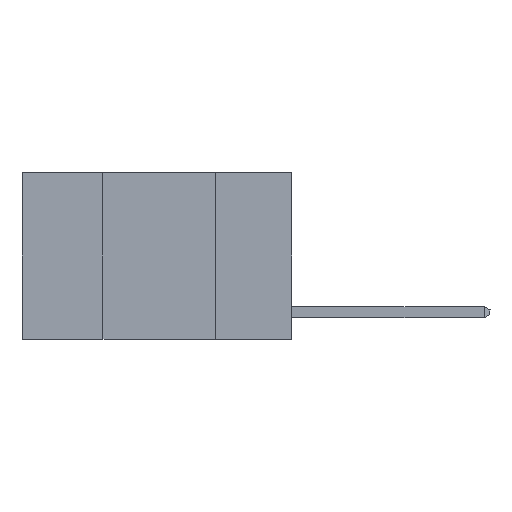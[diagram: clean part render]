
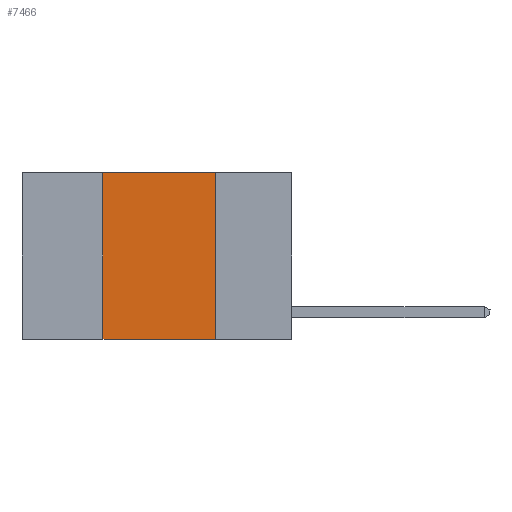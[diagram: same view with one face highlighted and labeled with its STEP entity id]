
A CAD part, left-side view. The second image highlights one B-rep face of the part: STEP entity #7466.
In plain terms, the highlighted planar face has unit normal (-1, 0, 0).
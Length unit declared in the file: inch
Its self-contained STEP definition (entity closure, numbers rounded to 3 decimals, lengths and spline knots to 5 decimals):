
#523 = CARTESIAN_POINT ( 'NONE',  ( 0., 0.42, -0.37 ) ) ;
#1208 = ORIENTED_EDGE ( 'NONE', *, *, #2267, .F. ) ;
#1470 = CARTESIAN_POINT ( 'NONE',  ( 0., 0.42, 0. ) ) ;
#2267 = EDGE_CURVE ( 'NONE', #13954, #2272, #3091, .T. ) ;
#2272 = VERTEX_POINT ( 'NONE', #8284 ) ;
#2611 = LINE ( 'NONE', #10808, #8658 ) ;
#3091 = LINE ( 'NONE', #8448, #12381 ) ;
#4083 = LINE ( 'NONE', #4106, #10171 ) ;
#4106 = CARTESIAN_POINT ( 'NONE',  ( 0., 0.42, 0. ) ) ;
#4417 = ORIENTED_EDGE ( 'NONE', *, *, #9108, .F. ) ;
#4813 = VECTOR ( 'NONE', #14393, 39.37008 ) ;
#4886 = DIRECTION ( 'NONE',  ( 0., 0., -1. ) ) ;
#5337 = DIRECTION ( 'NONE',  ( 0., 0., 1. ) ) ;
#5832 = CARTESIAN_POINT ( 'NONE',  ( 0., 0.17, -0.37 ) ) ;
#6704 = AXIS2_PLACEMENT_3D ( 'NONE', #9728, #12150, #4886 ) ;
#7096 = CARTESIAN_POINT ( 'NONE',  ( 0., 0.6, -0.37 ) ) ;
#7266 = PLANE ( 'NONE',  #6704 ) ;
#7336 = VERTEX_POINT ( 'NONE', #5832 ) ;
#7466 = ADVANCED_FACE ( 'NONE', ( #11537 ), #7266, .F. ) ;
#7810 = EDGE_LOOP ( 'NONE', ( #10499, #1208, #4417, #14109 ) ) ;
#8284 = CARTESIAN_POINT ( 'NONE',  ( 0., 0.17, 0. ) ) ;
#8317 = VERTEX_POINT ( 'NONE', #523 ) ;
#8444 = DIRECTION ( 'NONE',  ( 0., -1., 0. ) ) ;
#8448 = CARTESIAN_POINT ( 'NONE',  ( 0., 0.6, 0. ) ) ;
#8658 = VECTOR ( 'NONE', #12027, 39.37008 ) ;
#8804 = EDGE_CURVE ( 'NONE', #2272, #7336, #2611, .T. ) ;
#9108 = EDGE_CURVE ( 'NONE', #8317, #13954, #4083, .T. ) ;
#9728 = CARTESIAN_POINT ( 'NONE',  ( 0., 0.6, 0. ) ) ;
#10171 = VECTOR ( 'NONE', #5337, 39.37008 ) ;
#10499 = ORIENTED_EDGE ( 'NONE', *, *, #8804, .F. ) ;
#10808 = CARTESIAN_POINT ( 'NONE',  ( 0., 0.17, 0. ) ) ;
#11537 = FACE_OUTER_BOUND ( 'NONE', #7810, .T. ) ;
#12027 = DIRECTION ( 'NONE',  ( 0., 0., -1. ) ) ;
#12150 = DIRECTION ( 'NONE',  ( 1., 0., 0. ) ) ;
#12381 = VECTOR ( 'NONE', #8444, 39.37008 ) ;
#13063 = EDGE_CURVE ( 'NONE', #8317, #7336, #14507, .T. ) ;
#13954 = VERTEX_POINT ( 'NONE', #1470 ) ;
#14109 = ORIENTED_EDGE ( 'NONE', *, *, #13063, .T. ) ;
#14393 = DIRECTION ( 'NONE',  ( 0., -1., 0. ) ) ;
#14507 = LINE ( 'NONE', #7096, #4813 ) ;
